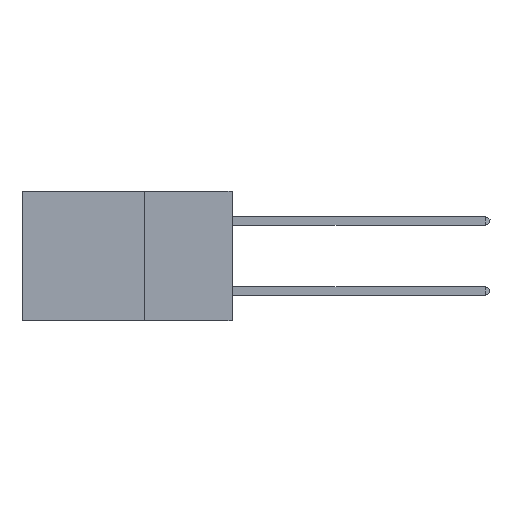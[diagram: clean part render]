
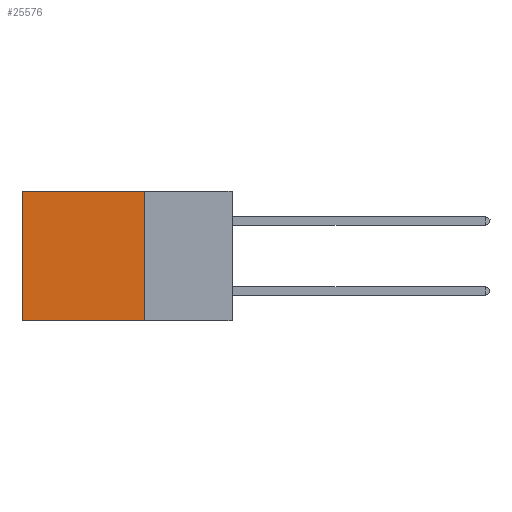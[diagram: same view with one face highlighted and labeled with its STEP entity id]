
A CAD part, left-side view. The second image highlights one B-rep face of the part: STEP entity #25576.
In plain terms, the highlighted planar face has unit normal (-1, 0, 0).
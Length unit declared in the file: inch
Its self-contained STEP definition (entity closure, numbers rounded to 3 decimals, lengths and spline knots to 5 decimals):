
#1038 = LINE ( 'NONE', #41535, #11106 ) ;
#1225 = VERTEX_POINT ( 'NONE', #28556 ) ;
#1628 = FACE_OUTER_BOUND ( 'NONE', #19326, .T. ) ;
#2734 = CARTESIAN_POINT ( 'NONE',  ( 0.2875, 0.25, -0.37 ) ) ;
#6025 = ORIENTED_EDGE ( 'NONE', *, *, #9095, .F. ) ;
#6537 = DIRECTION ( 'NONE',  ( 0., 1., 0. ) ) ;
#7235 = VERTEX_POINT ( 'NONE', #42263 ) ;
#7932 = ORIENTED_EDGE ( 'NONE', *, *, #16753, .T. ) ;
#9095 = EDGE_CURVE ( 'NONE', #7235, #16026, #1038, .T. ) ;
#10864 = VECTOR ( 'NONE', #26558, 39.37008 ) ;
#10971 = ORIENTED_EDGE ( 'NONE', *, *, #14901, .F. ) ;
#11106 = VECTOR ( 'NONE', #44983, 39.37008 ) ;
#14875 = DIRECTION ( 'NONE',  ( 1., 0., 0. ) ) ;
#14901 = EDGE_CURVE ( 'NONE', #16026, #1225, #26162, .T. ) ;
#16026 = VERTEX_POINT ( 'NONE', #42048 ) ;
#16753 = EDGE_CURVE ( 'NONE', #27428, #1225, #44425, .T. ) ;
#19326 = EDGE_LOOP ( 'NONE', ( #7932, #10971, #6025, #19455 ) ) ;
#19455 = ORIENTED_EDGE ( 'NONE', *, *, #23090, .T. ) ;
#21661 = DIRECTION ( 'NONE',  ( 0., 0., -1. ) ) ;
#22967 = CARTESIAN_POINT ( 'NONE',  ( 0.2875, 0.25, 0. ) ) ;
#23090 = EDGE_CURVE ( 'NONE', #7235, #27428, #29975, .T. ) ;
#24965 = CARTESIAN_POINT ( 'NONE',  ( 0.2875, 0.6, 0. ) ) ;
#25576 = ADVANCED_FACE ( 'NONE', ( #1628 ), #32455, .F. ) ;
#26162 = LINE ( 'NONE', #2734, #43527 ) ;
#26558 = DIRECTION ( 'NONE',  ( 0., 1., 0. ) ) ;
#27428 = VERTEX_POINT ( 'NONE', #24965 ) ;
#28556 = CARTESIAN_POINT ( 'NONE',  ( 0.2875, 0.6, -0.37 ) ) ;
#29113 = CARTESIAN_POINT ( 'NONE',  ( 0.2875, 0.25, 0. ) ) ;
#29975 = LINE ( 'NONE', #22967, #10864 ) ;
#32455 = PLANE ( 'NONE',  #40875 ) ;
#39154 = CARTESIAN_POINT ( 'NONE',  ( 0.2875, 0.6, 0. ) ) ;
#39592 = DIRECTION ( 'NONE',  ( 0., 0., -1. ) ) ;
#40875 = AXIS2_PLACEMENT_3D ( 'NONE', #29113, #14875, #39592 ) ;
#41535 = CARTESIAN_POINT ( 'NONE',  ( 0.2875, 0.25, 0. ) ) ;
#42048 = CARTESIAN_POINT ( 'NONE',  ( 0.2875, 0.25, -0.37 ) ) ;
#42263 = CARTESIAN_POINT ( 'NONE',  ( 0.2875, 0.25, 0. ) ) ;
#43349 = VECTOR ( 'NONE', #21661, 39.37008 ) ;
#43527 = VECTOR ( 'NONE', #6537, 39.37008 ) ;
#44425 = LINE ( 'NONE', #39154, #43349 ) ;
#44983 = DIRECTION ( 'NONE',  ( 0., 0., -1. ) ) ;
